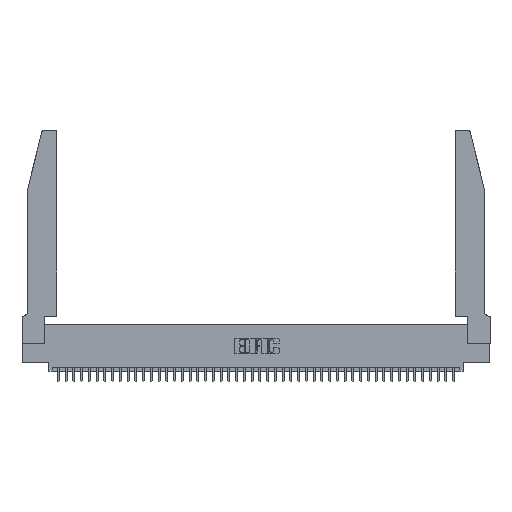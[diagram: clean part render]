
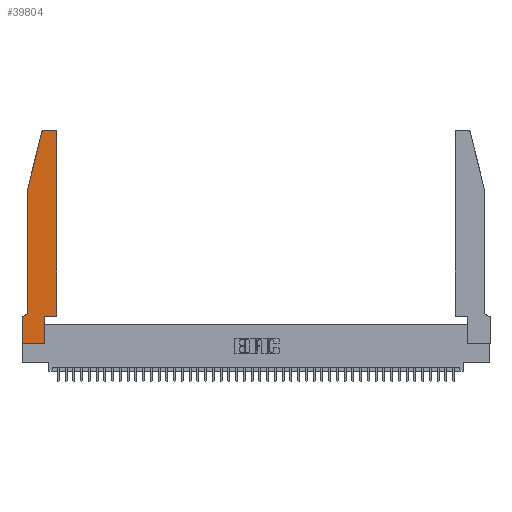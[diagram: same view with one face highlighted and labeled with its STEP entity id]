
A CAD part, top view. The second image highlights one B-rep face of the part: STEP entity #39804.
In plain terms, the highlighted planar face has unit normal (0, 0, 1).
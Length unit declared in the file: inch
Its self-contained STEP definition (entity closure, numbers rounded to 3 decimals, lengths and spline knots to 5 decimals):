
#78 = FACE_OUTER_BOUND ( 'NONE', #24696, .T. ) ;
#552 = ORIENTED_EDGE ( 'NONE', *, *, #25356, .T. ) ;
#604 = LINE ( 'NONE', #1570, #27061 ) ;
#729 = EDGE_CURVE ( 'NONE', #10550, #31738, #21457, .T. ) ;
#813 = EDGE_CURVE ( 'NONE', #27879, #10550, #44268, .T. ) ;
#982 = DIRECTION ( 'NONE',  ( -1., 0., 0. ) ) ;
#1174 = CARTESIAN_POINT ( 'NONE',  ( 0.284, 2.75, 0.37 ) ) ;
#1258 = CIRCLE ( 'NONE', #30793, 0.07 ) ;
#1570 = CARTESIAN_POINT ( 'NONE',  ( 0.4505, 0.35, 0.37 ) ) ;
#1875 = EDGE_CURVE ( 'NONE', #13556, #23066, #33023, .T. ) ;
#1906 = DIRECTION ( 'NONE',  ( 0., -1., 0. ) ) ;
#2739 = CARTESIAN_POINT ( 'NONE',  ( 0.4205, 2.75, 0.37 ) ) ;
#3022 = EDGE_CURVE ( 'NONE', #31738, #3549, #43541, .T. ) ;
#3549 = VERTEX_POINT ( 'NONE', #13041 ) ;
#4297 = VECTOR ( 'NONE', #982, 39.37008 ) ;
#4404 = VECTOR ( 'NONE', #8475, 39.37008 ) ;
#4763 = ORIENTED_EDGE ( 'NONE', *, *, #3022, .T. ) ;
#5583 = DIRECTION ( 'NONE',  ( 0., 0., 1. ) ) ;
#5761 = VERTEX_POINT ( 'NONE', #13800 ) ;
#6035 = ORIENTED_EDGE ( 'NONE', *, *, #34696, .T. ) ;
#6298 = DIRECTION ( 'NONE',  ( 0., 1., 0. ) ) ;
#6728 = CARTESIAN_POINT ( 'NONE',  ( 0.284, 2.72, 0.37 ) ) ;
#7240 = LINE ( 'NONE', #43602, #23359 ) ;
#7260 = VECTOR ( 'NONE', #34202, 39.37008 ) ;
#8475 = DIRECTION ( 'NONE',  ( 0., -1., 0. ) ) ;
#9231 = DIRECTION ( 'NONE',  ( 1., 0., 0. ) ) ;
#9476 = CARTESIAN_POINT ( 'NONE',  ( 0., 0., 0.37 ) ) ;
#10248 = DIRECTION ( 'NONE',  ( 1., 0., 0. ) ) ;
#10504 = VERTEX_POINT ( 'NONE', #43254 ) ;
#10550 = VERTEX_POINT ( 'NONE', #9476 ) ;
#11088 = ORIENTED_EDGE ( 'NONE', *, *, #41734, .T. ) ;
#11208 = ORIENTED_EDGE ( 'NONE', *, *, #27366, .T. ) ;
#11212 = AXIS2_PLACEMENT_3D ( 'NONE', #26246, #29692, #9231 ) ;
#13041 = CARTESIAN_POINT ( 'NONE',  ( 0.2865, 0.35, 0.37 ) ) ;
#13058 = VERTEX_POINT ( 'NONE', #1174 ) ;
#13247 = CARTESIAN_POINT ( 'NONE',  ( 0., 0.35, 0.37 ) ) ;
#13556 = VERTEX_POINT ( 'NONE', #17701 ) ;
#13800 = CARTESIAN_POINT ( 'NONE',  ( 0.0755, 0.42, 0.37 ) ) ;
#13852 = CARTESIAN_POINT ( 'NONE',  ( 0.4505, 2.72, 0.37 ) ) ;
#13945 = VECTOR ( 'NONE', #37663, 39.37008 ) ;
#14257 = EDGE_CURVE ( 'NONE', #23066, #5761, #23831, .T. ) ;
#14953 = VECTOR ( 'NONE', #32173, 39.37008 ) ;
#15240 = CARTESIAN_POINT ( 'NONE',  ( 0.0755, 2., 0.37 ) ) ;
#15265 = AXIS2_PLACEMENT_3D ( 'NONE', #6728, #30675, #10248 ) ;
#17182 = VECTOR ( 'NONE', #1906, 39.37008 ) ;
#17701 = CARTESIAN_POINT ( 'NONE',  ( 0.25487, 2.72718, 0.37 ) ) ;
#18297 = CARTESIAN_POINT ( 'NONE',  ( 0.2605, 2.75, 0.37 ) ) ;
#20462 = CARTESIAN_POINT ( 'NONE',  ( 0.0055, 0.42, 0.37 ) ) ;
#20543 = CARTESIAN_POINT ( 'NONE',  ( 0.2865, 0.35, 0.37 ) ) ;
#20746 = CARTESIAN_POINT ( 'NONE',  ( 0.0755, 0.35, 0.37 ) ) ;
#21457 = LINE ( 'NONE', #42503, #38423 ) ;
#22777 = CARTESIAN_POINT ( 'NONE',  ( 0.0755, 2., 0.37 ) ) ;
#22859 = PLANE ( 'NONE',  #11212 ) ;
#23066 = VERTEX_POINT ( 'NONE', #22777 ) ;
#23359 = VECTOR ( 'NONE', #6298, 39.37008 ) ;
#23494 = ORIENTED_EDGE ( 'NONE', *, *, #39893, .T. ) ;
#23831 = LINE ( 'NONE', #25531, #4404 ) ;
#23887 = DIRECTION ( 'NONE',  ( -1., 0., 0. ) ) ;
#24340 = ORIENTED_EDGE ( 'NONE', *, *, #1875, .T. ) ;
#24696 = EDGE_LOOP ( 'NONE', ( #552, #11088, #24340, #27782, #6035, #11208, #33714, #29720, #4763, #40947, #23494, #39218 ) ) ;
#25356 = EDGE_CURVE ( 'NONE', #36839, #13058, #41773, .T. ) ;
#25531 = CARTESIAN_POINT ( 'NONE',  ( 0.0755, 2., 0.37 ) ) ;
#25710 = DIRECTION ( 'NONE',  ( 1., 0., 0. ) ) ;
#25948 = AXIS2_PLACEMENT_3D ( 'NONE', #26142, #5583, #29590 ) ;
#26142 = CARTESIAN_POINT ( 'NONE',  ( 0.4205, 2.72, 0.37 ) ) ;
#26246 = CARTESIAN_POINT ( 'NONE',  ( 0., 0.35, 0.37 ) ) ;
#26996 = CARTESIAN_POINT ( 'NONE',  ( 0.4505, 0.35, 0.37 ) ) ;
#27061 = VECTOR ( 'NONE', #25710, 39.37008 ) ;
#27366 = EDGE_CURVE ( 'NONE', #10504, #27879, #33078, .T. ) ;
#27782 = ORIENTED_EDGE ( 'NONE', *, *, #14257, .T. ) ;
#27879 = VERTEX_POINT ( 'NONE', #13247 ) ;
#29026 = DIRECTION ( 'NONE',  ( 1., 0., 0. ) ) ;
#29590 = DIRECTION ( 'NONE',  ( 1., 0., 0. ) ) ;
#29692 = DIRECTION ( 'NONE',  ( 0., 0., 1. ) ) ;
#29720 = ORIENTED_EDGE ( 'NONE', *, *, #729, .T. ) ;
#30675 = DIRECTION ( 'NONE',  ( 0., 0., 1. ) ) ;
#30793 = AXIS2_PLACEMENT_3D ( 'NONE', #20462, #44194, #23887 ) ;
#31140 = CIRCLE ( 'NONE', #15265, 0.03 ) ;
#31738 = VERTEX_POINT ( 'NONE', #34464 ) ;
#32173 = DIRECTION ( 'NONE',  ( -0.239, -0.971, 0. ) ) ;
#33023 = LINE ( 'NONE', #15240, #14953 ) ;
#33078 = LINE ( 'NONE', #20746, #13945 ) ;
#33714 = ORIENTED_EDGE ( 'NONE', *, *, #813, .T. ) ;
#34202 = DIRECTION ( 'NONE',  ( 0., 1., 0. ) ) ;
#34464 = CARTESIAN_POINT ( 'NONE',  ( 0.2865, 0., 0.37 ) ) ;
#34676 = VERTEX_POINT ( 'NONE', #26996 ) ;
#34696 = EDGE_CURVE ( 'NONE', #5761, #10504, #1258, .T. ) ;
#35401 = VERTEX_POINT ( 'NONE', #13852 ) ;
#35839 = EDGE_CURVE ( 'NONE', #3549, #34676, #604, .T. ) ;
#35929 = EDGE_CURVE ( 'NONE', #35401, #36839, #40862, .T. ) ;
#36839 = VERTEX_POINT ( 'NONE', #2739 ) ;
#37663 = DIRECTION ( 'NONE',  ( -1., 0., 0. ) ) ;
#38423 = VECTOR ( 'NONE', #29026, 39.37008 ) ;
#39218 = ORIENTED_EDGE ( 'NONE', *, *, #35929, .T. ) ;
#39804 = ADVANCED_FACE ( 'NONE', ( #78 ), #22859, .T. ) ;
#39893 = EDGE_CURVE ( 'NONE', #34676, #35401, #7240, .T. ) ;
#40862 = CIRCLE ( 'NONE', #25948, 0.03 ) ;
#40947 = ORIENTED_EDGE ( 'NONE', *, *, #35839, .T. ) ;
#41734 = EDGE_CURVE ( 'NONE', #13058, #13556, #31140, .T. ) ;
#41773 = LINE ( 'NONE', #18297, #4297 ) ;
#42503 = CARTESIAN_POINT ( 'NONE',  ( 0., 0., 0.37 ) ) ;
#42939 = CARTESIAN_POINT ( 'NONE',  ( 0., 0., 0.37 ) ) ;
#43254 = CARTESIAN_POINT ( 'NONE',  ( 0.0055, 0.35, 0.37 ) ) ;
#43541 = LINE ( 'NONE', #20543, #7260 ) ;
#43602 = CARTESIAN_POINT ( 'NONE',  ( 0.4505, 0.35, 0.37 ) ) ;
#44194 = DIRECTION ( 'NONE',  ( 0., 0., -1. ) ) ;
#44268 = LINE ( 'NONE', #42939, #17182 ) ;
